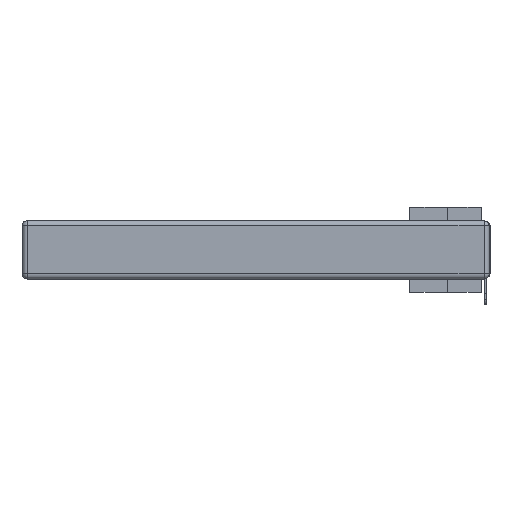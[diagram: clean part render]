
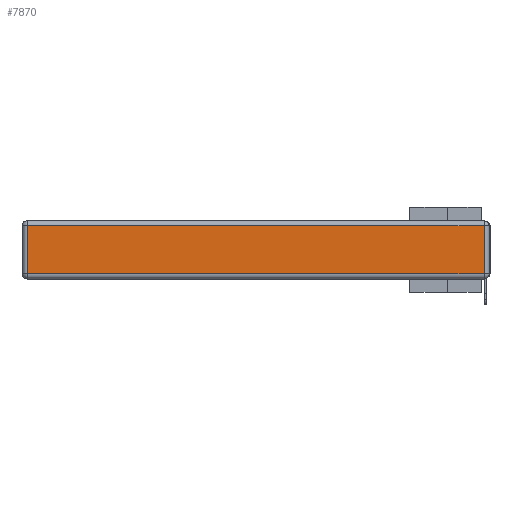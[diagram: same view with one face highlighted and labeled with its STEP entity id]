
A CAD part, left-side view. The second image highlights one B-rep face of the part: STEP entity #7870.
In plain terms, the highlighted planar face has unit normal (-1, 0, 0).
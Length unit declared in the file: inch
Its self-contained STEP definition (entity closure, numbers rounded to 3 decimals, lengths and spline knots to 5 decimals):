
#303 = CARTESIAN_POINT ( 'NONE',  ( 0., 0.03, -0.313 ) ) ;
#3228 = VECTOR ( 'NONE', #27100, 39.37008 ) ;
#5004 = EDGE_CURVE ( 'NONE', #6369, #36901, #31174, .T. ) ;
#5478 = VECTOR ( 'NONE', #18795, 39.37008 ) ;
#5919 = FACE_OUTER_BOUND ( 'NONE', #12580, .T. ) ;
#6062 = ORIENTED_EDGE ( 'NONE', *, *, #30683, .T. ) ;
#6369 = VERTEX_POINT ( 'NONE', #37811 ) ;
#6902 = CARTESIAN_POINT ( 'NONE',  ( 0., 2.72, -0.313 ) ) ;
#6985 = CARTESIAN_POINT ( 'NONE',  ( 0., 0.03, -0.03 ) ) ;
#6994 = EDGE_CURVE ( 'NONE', #36901, #31000, #15283, .T. ) ;
#7870 = ADVANCED_FACE ( 'NONE', ( #5919 ), #12104, .T. ) ;
#10580 = DIRECTION ( 'NONE',  ( 0., 1., 0. ) ) ;
#10728 = VERTEX_POINT ( 'NONE', #6985 ) ;
#12104 = PLANE ( 'NONE',  #32849 ) ;
#12580 = EDGE_LOOP ( 'NONE', ( #31271, #19851, #6062, #25513 ) ) ;
#13276 = CARTESIAN_POINT ( 'NONE',  ( 0., 2.75, -0.03 ) ) ;
#14612 = CARTESIAN_POINT ( 'NONE',  ( 0., 0., -0.343 ) ) ;
#15283 = LINE ( 'NONE', #26331, #3228 ) ;
#18795 = DIRECTION ( 'NONE',  ( 0., 0., -1. ) ) ;
#19851 = ORIENTED_EDGE ( 'NONE', *, *, #31294, .T. ) ;
#20006 = LINE ( 'NONE', #20204, #31207 ) ;
#20204 = CARTESIAN_POINT ( 'NONE',  ( 0., 0.03, -0.343 ) ) ;
#20399 = DIRECTION ( 'NONE',  ( 0., 0., 1. ) ) ;
#22008 = LINE ( 'NONE', #13276, #28093 ) ;
#23150 = DIRECTION ( 'NONE',  ( -1., 0., 0. ) ) ;
#23727 = DIRECTION ( 'NONE',  ( 0., 0., 1. ) ) ;
#25513 = ORIENTED_EDGE ( 'NONE', *, *, #5004, .T. ) ;
#26331 = CARTESIAN_POINT ( 'NONE',  ( 0., 0., -0.313 ) ) ;
#27100 = DIRECTION ( 'NONE',  ( 0., -1., 0. ) ) ;
#27712 = CARTESIAN_POINT ( 'NONE',  ( 0., 2.72, -0.343 ) ) ;
#28093 = VECTOR ( 'NONE', #10580, 39.37008 ) ;
#30683 = EDGE_CURVE ( 'NONE', #10728, #6369, #22008, .T. ) ;
#31000 = VERTEX_POINT ( 'NONE', #303 ) ;
#31174 = LINE ( 'NONE', #27712, #5478 ) ;
#31207 = VECTOR ( 'NONE', #20399, 39.37008 ) ;
#31271 = ORIENTED_EDGE ( 'NONE', *, *, #6994, .T. ) ;
#31294 = EDGE_CURVE ( 'NONE', #31000, #10728, #20006, .T. ) ;
#32849 = AXIS2_PLACEMENT_3D ( 'NONE', #14612, #23150, #23727 ) ;
#36901 = VERTEX_POINT ( 'NONE', #6902 ) ;
#37811 = CARTESIAN_POINT ( 'NONE',  ( 0., 2.72, -0.03 ) ) ;
